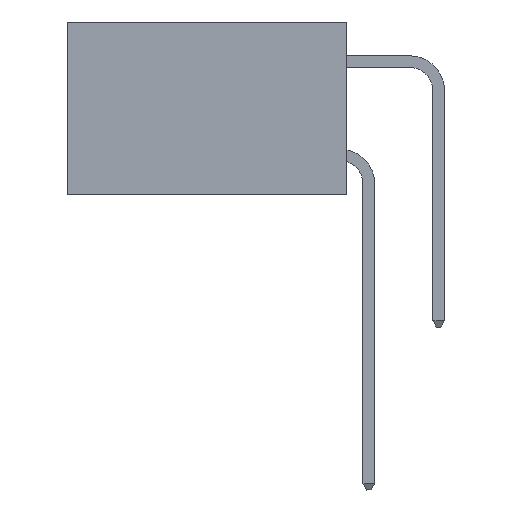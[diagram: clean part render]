
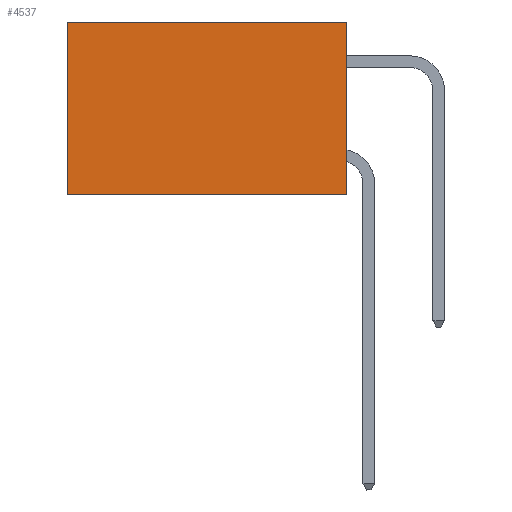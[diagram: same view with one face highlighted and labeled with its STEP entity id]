
A CAD part, left-side view. The second image highlights one B-rep face of the part: STEP entity #4537.
In plain terms, the highlighted planar face has unit normal (-1, 0, 0).
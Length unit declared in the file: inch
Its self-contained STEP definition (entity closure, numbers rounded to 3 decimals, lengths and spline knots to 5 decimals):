
#826 = DIRECTION ( 'NONE',  ( 0., 0., -1. ) ) ;
#1128 = DIRECTION ( 'NONE',  ( 0., 1., 0. ) ) ;
#1659 = VECTOR ( 'NONE', #826, 39.37008 ) ;
#1859 = LINE ( 'NONE', #21541, #21577 ) ;
#2053 = ORIENTED_EDGE ( 'NONE', *, *, #6681, .T. ) ;
#2124 = DIRECTION ( 'NONE',  ( 1., 0., 0. ) ) ;
#2157 = DIRECTION ( 'NONE',  ( 0., 0., -1. ) ) ;
#2314 = PLANE ( 'NONE',  #9986 ) ;
#2343 = CARTESIAN_POINT ( 'NONE',  ( 0.2875, 0., 0. ) ) ;
#2381 = ORIENTED_EDGE ( 'NONE', *, *, #18987, .F. ) ;
#2581 = CARTESIAN_POINT ( 'NONE',  ( 0.2875, 0., 0. ) ) ;
#2876 = CARTESIAN_POINT ( 'NONE',  ( 0.2875, 0., 0. ) ) ;
#3023 = VERTEX_POINT ( 'NONE', #19555 ) ;
#4024 = VERTEX_POINT ( 'NONE', #7642 ) ;
#4537 = ADVANCED_FACE ( 'NONE', ( #14887 ), #2314, .F. ) ;
#4775 = CARTESIAN_POINT ( 'NONE',  ( 0.2875, 0.6, 0. ) ) ;
#5284 = DIRECTION ( 'NONE',  ( 0., 1., 0. ) ) ;
#5966 = EDGE_CURVE ( 'NONE', #16445, #4024, #21941, .T. ) ;
#6681 = EDGE_CURVE ( 'NONE', #3023, #16445, #21637, .T. ) ;
#6828 = LINE ( 'NONE', #2876, #1659 ) ;
#7628 = DIRECTION ( 'NONE',  ( 0., 0., -1. ) ) ;
#7642 = CARTESIAN_POINT ( 'NONE',  ( 0.2875, 0.6, -0.37 ) ) ;
#8289 = VECTOR ( 'NONE', #5284, 39.37008 ) ;
#8896 = ORIENTED_EDGE ( 'NONE', *, *, #5966, .T. ) ;
#9986 = AXIS2_PLACEMENT_3D ( 'NONE', #2343, #2124, #2157 ) ;
#10176 = ORIENTED_EDGE ( 'NONE', *, *, #16453, .F. ) ;
#11711 = CARTESIAN_POINT ( 'NONE',  ( 0.2875, 0.6, 0. ) ) ;
#14887 = FACE_OUTER_BOUND ( 'NONE', #19521, .T. ) ;
#15226 = CARTESIAN_POINT ( 'NONE',  ( 0.2875, 0., -0.37 ) ) ;
#16445 = VERTEX_POINT ( 'NONE', #4775 ) ;
#16453 = EDGE_CURVE ( 'NONE', #3023, #18624, #6828, .T. ) ;
#18624 = VERTEX_POINT ( 'NONE', #15226 ) ;
#18987 = EDGE_CURVE ( 'NONE', #18624, #4024, #1859, .T. ) ;
#19521 = EDGE_LOOP ( 'NONE', ( #8896, #2381, #10176, #2053 ) ) ;
#19555 = CARTESIAN_POINT ( 'NONE',  ( 0.2875, 0., 0. ) ) ;
#21379 = VECTOR ( 'NONE', #7628, 39.37008 ) ;
#21541 = CARTESIAN_POINT ( 'NONE',  ( 0.2875, 0., -0.37 ) ) ;
#21577 = VECTOR ( 'NONE', #1128, 39.37008 ) ;
#21637 = LINE ( 'NONE', #2581, #8289 ) ;
#21941 = LINE ( 'NONE', #11711, #21379 ) ;
